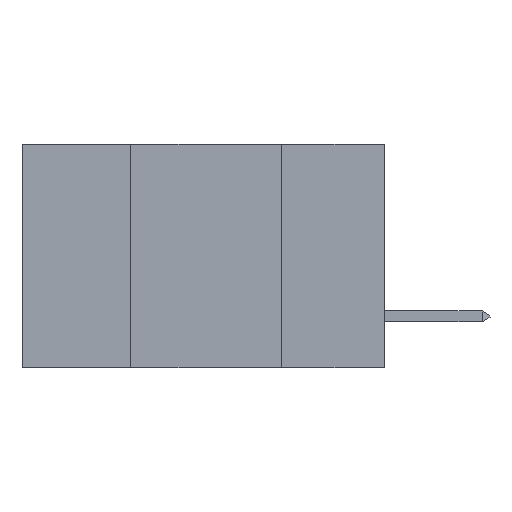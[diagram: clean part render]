
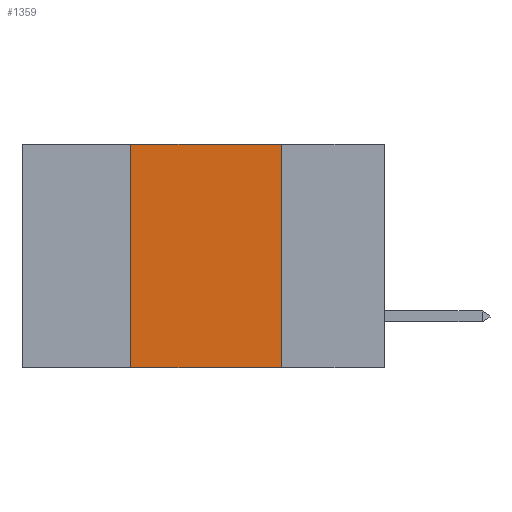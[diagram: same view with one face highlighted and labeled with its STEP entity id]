
A CAD part, left-side view. The second image highlights one B-rep face of the part: STEP entity #1359.
In plain terms, the highlighted planar face has unit normal (-1, 0, 0).
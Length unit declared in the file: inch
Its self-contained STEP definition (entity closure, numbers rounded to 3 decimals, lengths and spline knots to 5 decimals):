
#250 = CARTESIAN_POINT ( 'NONE',  ( 0., 0.42, -0.37 ) ) ;
#1359 = ADVANCED_FACE ( 'NONE', ( #20679 ), #8307, .F. ) ;
#1532 = LINE ( 'NONE', #27482, #7767 ) ;
#3209 = VECTOR ( 'NONE', #28687, 39.37008 ) ;
#3290 = ORIENTED_EDGE ( 'NONE', *, *, #5401, .T. ) ;
#3295 = VERTEX_POINT ( 'NONE', #25612 ) ;
#3931 = LINE ( 'NONE', #14560, #3209 ) ;
#5401 = EDGE_CURVE ( 'NONE', #11917, #26364, #29199, .T. ) ;
#5530 = EDGE_LOOP ( 'NONE', ( #24040, #19965, #10406, #3290 ) ) ;
#5688 = VERTEX_POINT ( 'NONE', #10535 ) ;
#6882 = CARTESIAN_POINT ( 'NONE',  ( 0., 0.42, 0. ) ) ;
#7767 = VECTOR ( 'NONE', #29818, 39.37008 ) ;
#7771 = DIRECTION ( 'NONE',  ( 0., 0., -1. ) ) ;
#7826 = DIRECTION ( 'NONE',  ( 1., 0., 0. ) ) ;
#7970 = CARTESIAN_POINT ( 'NONE',  ( 0., 0.6, 0. ) ) ;
#8307 = PLANE ( 'NONE',  #27540 ) ;
#9267 = VECTOR ( 'NONE', #28312, 39.37008 ) ;
#10406 = ORIENTED_EDGE ( 'NONE', *, *, #15075, .F. ) ;
#10535 = CARTESIAN_POINT ( 'NONE',  ( 0., 0.42, 0. ) ) ;
#11917 = VERTEX_POINT ( 'NONE', #250 ) ;
#13245 = CARTESIAN_POINT ( 'NONE',  ( 0., 0.17, -0.37 ) ) ;
#14560 = CARTESIAN_POINT ( 'NONE',  ( 0., 0.17, 0. ) ) ;
#15075 = EDGE_CURVE ( 'NONE', #11917, #5688, #28239, .T. ) ;
#19145 = CARTESIAN_POINT ( 'NONE',  ( 0., 0.6, -0.37 ) ) ;
#19965 = ORIENTED_EDGE ( 'NONE', *, *, #29001, .F. ) ;
#20679 = FACE_OUTER_BOUND ( 'NONE', #5530, .T. ) ;
#22294 = VECTOR ( 'NONE', #23926, 39.37008 ) ;
#23926 = DIRECTION ( 'NONE',  ( 0., -1., 0. ) ) ;
#24040 = ORIENTED_EDGE ( 'NONE', *, *, #25454, .F. ) ;
#25454 = EDGE_CURVE ( 'NONE', #3295, #26364, #3931, .T. ) ;
#25612 = CARTESIAN_POINT ( 'NONE',  ( 0., 0.17, 0. ) ) ;
#26364 = VERTEX_POINT ( 'NONE', #13245 ) ;
#27482 = CARTESIAN_POINT ( 'NONE',  ( 0., 0.6, 0. ) ) ;
#27540 = AXIS2_PLACEMENT_3D ( 'NONE', #7970, #7826, #7771 ) ;
#28239 = LINE ( 'NONE', #6882, #9267 ) ;
#28312 = DIRECTION ( 'NONE',  ( 0., 0., 1. ) ) ;
#28687 = DIRECTION ( 'NONE',  ( 0., 0., -1. ) ) ;
#29001 = EDGE_CURVE ( 'NONE', #5688, #3295, #1532, .T. ) ;
#29199 = LINE ( 'NONE', #19145, #22294 ) ;
#29818 = DIRECTION ( 'NONE',  ( 0., -1., 0. ) ) ;
